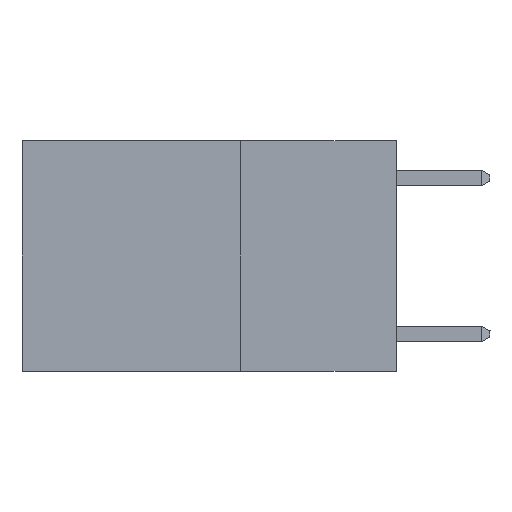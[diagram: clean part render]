
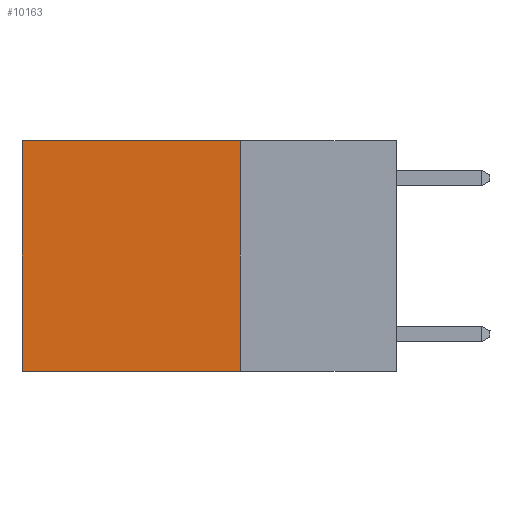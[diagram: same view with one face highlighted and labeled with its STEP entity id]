
A CAD part, left-side view. The second image highlights one B-rep face of the part: STEP entity #10163.
In plain terms, the highlighted planar face has unit normal (-1, 0, 0).
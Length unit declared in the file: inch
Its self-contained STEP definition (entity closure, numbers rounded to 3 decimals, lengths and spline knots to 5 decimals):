
#847 = LINE ( 'NONE', #7553, #8444 ) ;
#1150 = VECTOR ( 'NONE', #11027, 39.37008 ) ;
#1520 = LINE ( 'NONE', #2530, #3919 ) ;
#1634 = CARTESIAN_POINT ( 'NONE',  ( 0.2625, 0.6, 0. ) ) ;
#1832 = LINE ( 'NONE', #10077, #1150 ) ;
#2530 = CARTESIAN_POINT ( 'NONE',  ( 0.2625, 0.25, 0. ) ) ;
#3062 = CARTESIAN_POINT ( 'NONE',  ( 0.2625, 0.25, -0.37 ) ) ;
#3149 = ORIENTED_EDGE ( 'NONE', *, *, #11191, .F. ) ;
#3546 = DIRECTION ( 'NONE',  ( 0., 1., 0. ) ) ;
#3678 = DIRECTION ( 'NONE',  ( 0., 0., -1. ) ) ;
#3919 = VECTOR ( 'NONE', #3546, 39.37008 ) ;
#3979 = EDGE_LOOP ( 'NONE', ( #7807, #7263, #3149, #8480 ) ) ;
#4431 = VERTEX_POINT ( 'NONE', #5634 ) ;
#5337 = VERTEX_POINT ( 'NONE', #11957 ) ;
#5634 = CARTESIAN_POINT ( 'NONE',  ( 0.2625, 0.25, 0. ) ) ;
#6133 = EDGE_CURVE ( 'NONE', #12390, #5337, #10853, .T. ) ;
#6624 = DIRECTION ( 'NONE',  ( 0., 1., 0. ) ) ;
#6761 = DIRECTION ( 'NONE',  ( 1., 0., 0. ) ) ;
#7263 = ORIENTED_EDGE ( 'NONE', *, *, #9391, .F. ) ;
#7553 = CARTESIAN_POINT ( 'NONE',  ( 0.2625, 0.25, -0.37 ) ) ;
#7680 = CARTESIAN_POINT ( 'NONE',  ( 0.2625, 0.25, 0. ) ) ;
#7807 = ORIENTED_EDGE ( 'NONE', *, *, #6133, .T. ) ;
#7992 = VERTEX_POINT ( 'NONE', #3062 ) ;
#8338 = VECTOR ( 'NONE', #3678, 39.37008 ) ;
#8444 = VECTOR ( 'NONE', #6624, 39.37008 ) ;
#8480 = ORIENTED_EDGE ( 'NONE', *, *, #9955, .T. ) ;
#9391 = EDGE_CURVE ( 'NONE', #7992, #5337, #847, .T. ) ;
#9494 = FACE_OUTER_BOUND ( 'NONE', #3979, .T. ) ;
#9636 = PLANE ( 'NONE',  #10898 ) ;
#9955 = EDGE_CURVE ( 'NONE', #4431, #12390, #1520, .T. ) ;
#10077 = CARTESIAN_POINT ( 'NONE',  ( 0.2625, 0.25, 0. ) ) ;
#10163 = ADVANCED_FACE ( 'NONE', ( #9494 ), #9636, .F. ) ;
#10853 = LINE ( 'NONE', #1634, #8338 ) ;
#10898 = AXIS2_PLACEMENT_3D ( 'NONE', #7680, #6761, #11636 ) ;
#11027 = DIRECTION ( 'NONE',  ( 0., 0., -1. ) ) ;
#11191 = EDGE_CURVE ( 'NONE', #4431, #7992, #1832, .T. ) ;
#11446 = CARTESIAN_POINT ( 'NONE',  ( 0.2625, 0.6, 0. ) ) ;
#11636 = DIRECTION ( 'NONE',  ( 0., 0., -1. ) ) ;
#11957 = CARTESIAN_POINT ( 'NONE',  ( 0.2625, 0.6, -0.37 ) ) ;
#12390 = VERTEX_POINT ( 'NONE', #11446 ) ;
